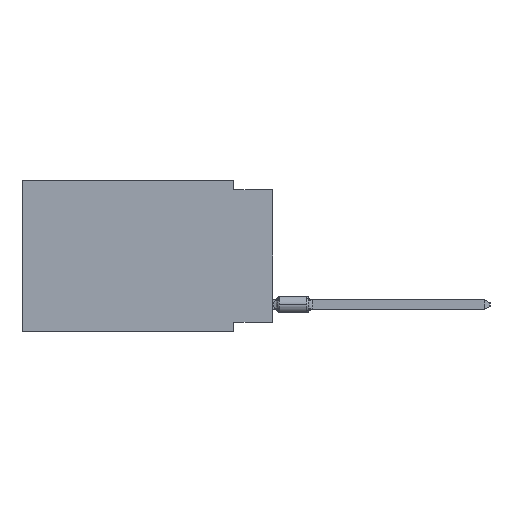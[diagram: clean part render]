
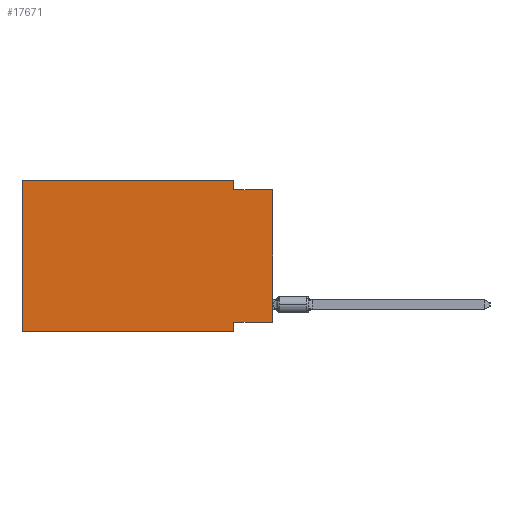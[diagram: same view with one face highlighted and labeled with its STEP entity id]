
A CAD part, left-side view. The second image highlights one B-rep face of the part: STEP entity #17671.
In plain terms, the highlighted planar face has unit normal (-1, 0, 0).
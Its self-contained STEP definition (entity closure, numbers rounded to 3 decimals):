
#870 = VECTOR ( 'NONE', #38791, 1000. ) ;
#1547 = VECTOR ( 'NONE', #22662, 1000. ) ;
#1683 = EDGE_CURVE ( 'NONE', #12937, #12145, #36830, .T. ) ;
#2987 = CARTESIAN_POINT ( 'NONE',  ( 0., 16.383, -9.906 ) ) ;
#3676 = DIRECTION ( 'NONE',  ( 0., -1., 0. ) ) ;
#3832 = VECTOR ( 'NONE', #21665, 1000. ) ;
#4053 = EDGE_LOOP ( 'NONE', ( #31061, #34747, #9463, #22734, #27365, #8893, #16743, #11813 ) ) ;
#4503 = CARTESIAN_POINT ( 'NONE',  ( 0., 0., -9.271 ) ) ;
#4914 = EDGE_CURVE ( 'NONE', #12402, #40044, #32076, .T. ) ;
#5120 = EDGE_CURVE ( 'NONE', #34637, #8227, #34435, .T. ) ;
#5408 = CARTESIAN_POINT ( 'NONE',  ( 0., 2.54, -9.271 ) ) ;
#5896 = EDGE_CURVE ( 'NONE', #14845, #40044, #33428, .T. ) ;
#6464 = VERTEX_POINT ( 'NONE', #23011 ) ;
#8227 = VERTEX_POINT ( 'NONE', #24990 ) ;
#8601 = CARTESIAN_POINT ( 'NONE',  ( 0., 16.383, 0. ) ) ;
#8893 = ORIENTED_EDGE ( 'NONE', *, *, #5896, .T. ) ;
#9389 = CARTESIAN_POINT ( 'NONE',  ( 0., 16.383, 0. ) ) ;
#9463 = ORIENTED_EDGE ( 'NONE', *, *, #5120, .F. ) ;
#9630 = AXIS2_PLACEMENT_3D ( 'NONE', #8601, #25354, #15967 ) ;
#10580 = VECTOR ( 'NONE', #3676, 1000. ) ;
#10775 = CARTESIAN_POINT ( 'NONE',  ( 0., 0., 0. ) ) ;
#11813 = ORIENTED_EDGE ( 'NONE', *, *, #12856, .F. ) ;
#12145 = VERTEX_POINT ( 'NONE', #19858 ) ;
#12402 = VERTEX_POINT ( 'NONE', #5408 ) ;
#12856 = EDGE_CURVE ( 'NONE', #12937, #12402, #34267, .T. ) ;
#12937 = VERTEX_POINT ( 'NONE', #29458 ) ;
#13761 = DIRECTION ( 'NONE',  ( 0., 0., 1. ) ) ;
#14845 = VERTEX_POINT ( 'NONE', #25466 ) ;
#15566 = CARTESIAN_POINT ( 'NONE',  ( 0., 2.54, -9.906 ) ) ;
#15967 = DIRECTION ( 'NONE',  ( 0., 0., -1. ) ) ;
#16743 = ORIENTED_EDGE ( 'NONE', *, *, #4914, .F. ) ;
#17671 = ADVANCED_FACE ( 'NONE', ( #22735 ), #32704, .F. ) ;
#18105 = CARTESIAN_POINT ( 'NONE',  ( 0., 2.54, 0. ) ) ;
#19858 = CARTESIAN_POINT ( 'NONE',  ( 0., 0., -0.635 ) ) ;
#21665 = DIRECTION ( 'NONE',  ( 0., 1., 0. ) ) ;
#22662 = DIRECTION ( 'NONE',  ( 0., -1., 0. ) ) ;
#22734 = ORIENTED_EDGE ( 'NONE', *, *, #26761, .F. ) ;
#22735 = FACE_OUTER_BOUND ( 'NONE', #4053, .T. ) ;
#23011 = CARTESIAN_POINT ( 'NONE',  ( 0., 16.383, 0. ) ) ;
#23862 = EDGE_CURVE ( 'NONE', #8227, #12145, #39323, .T. ) ;
#24873 = CARTESIAN_POINT ( 'NONE',  ( 0., 2.54, 0. ) ) ;
#24990 = CARTESIAN_POINT ( 'NONE',  ( 0., 2.54, -0.635 ) ) ;
#25354 = DIRECTION ( 'NONE',  ( 1., 0., 0. ) ) ;
#25466 = CARTESIAN_POINT ( 'NONE',  ( 0., 16.383, -9.906 ) ) ;
#25757 = VECTOR ( 'NONE', #37252, 1000. ) ;
#26761 = EDGE_CURVE ( 'NONE', #6464, #34637, #39126, .T. ) ;
#27365 = ORIENTED_EDGE ( 'NONE', *, *, #40187, .F. ) ;
#29364 = CARTESIAN_POINT ( 'NONE',  ( 0., 0., -0.635 ) ) ;
#29458 = CARTESIAN_POINT ( 'NONE',  ( 0., 0., -9.271 ) ) ;
#30070 = CARTESIAN_POINT ( 'NONE',  ( 0., 16.383, 0. ) ) ;
#31061 = ORIENTED_EDGE ( 'NONE', *, *, #1683, .T. ) ;
#31792 = VECTOR ( 'NONE', #13761, 1000. ) ;
#32076 = LINE ( 'NONE', #15566, #870 ) ;
#32704 = PLANE ( 'NONE',  #9630 ) ;
#33428 = LINE ( 'NONE', #2987, #10580 ) ;
#34267 = LINE ( 'NONE', #4503, #3832 ) ;
#34435 = LINE ( 'NONE', #24873, #35552 ) ;
#34637 = VERTEX_POINT ( 'NONE', #18105 ) ;
#34747 = ORIENTED_EDGE ( 'NONE', *, *, #23862, .F. ) ;
#35552 = VECTOR ( 'NONE', #41144, 1000. ) ;
#36830 = LINE ( 'NONE', #10775, #25757 ) ;
#37252 = DIRECTION ( 'NONE',  ( 0., 0., 1. ) ) ;
#38791 = DIRECTION ( 'NONE',  ( 0., 0., -1. ) ) ;
#39126 = LINE ( 'NONE', #9389, #1547 ) ;
#39323 = LINE ( 'NONE', #29364, #41979 ) ;
#39387 = LINE ( 'NONE', #30070, #31792 ) ;
#40044 = VERTEX_POINT ( 'NONE', #42660 ) ;
#40187 = EDGE_CURVE ( 'NONE', #14845, #6464, #39387, .T. ) ;
#41144 = DIRECTION ( 'NONE',  ( 0., 0., -1. ) ) ;
#41979 = VECTOR ( 'NONE', #42595, 1000. ) ;
#42595 = DIRECTION ( 'NONE',  ( 0., -1., 0. ) ) ;
#42660 = CARTESIAN_POINT ( 'NONE',  ( 0., 2.54, -9.906 ) ) ;
